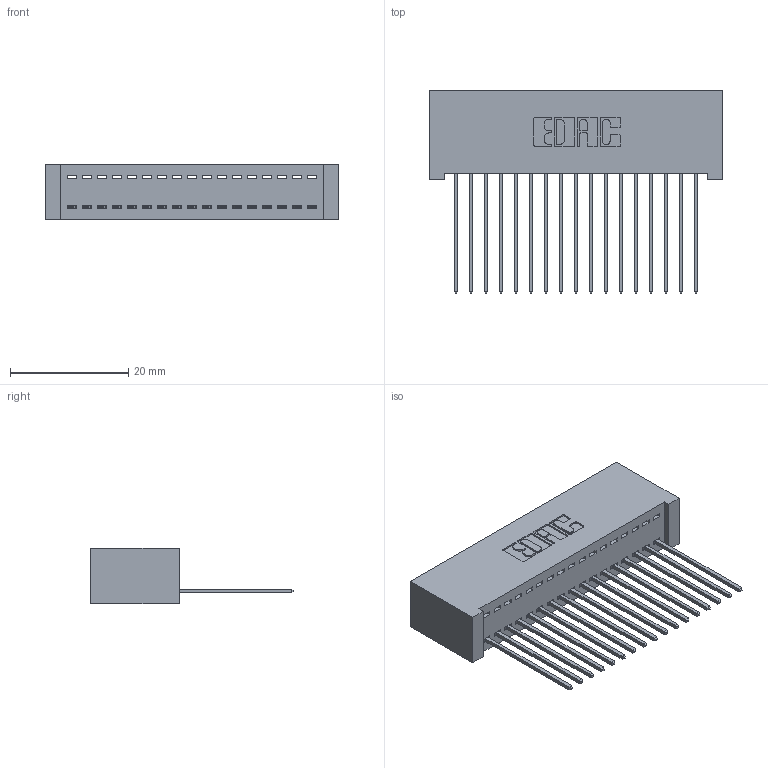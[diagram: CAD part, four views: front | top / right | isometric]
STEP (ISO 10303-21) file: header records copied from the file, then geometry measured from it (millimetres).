
FILE_DESCRIPTION (( 'STEP AP203' ), '1' );
FILE_NAME ('392-017-541-101.STEP', '2019-10-07T03:41:49', ( '' ), ( '' ), 'SwSTEP 2.0', 'SolidWorks 2016', '' );
FILE_SCHEMA (( 'CONFIG_CONTROL_DESIGN' ));
Length unit declared in the file: inch
Products named in the file (3): 342 Part_Lugless; 345-292-001_345-293-141; 392-017-541-101
Assembly tree (18 placements, depth 2):
  392-017-541-101
    342 Part_Lugless
    345-292-001_345-293-141  x17
Bounding box: 49.43 x 34.3 x 9.4 mm (x, y, z)
Volume: 4706.9 mm3; surface area: 7087.3 mm2
Topology: 18 solids, 18 shells, 1088 faces, 3267 edges, 2154 vertices
Faces by surface type: plane 776, cylinder 312
Entity records: 13235 total; most frequent: CARTESIAN_POINT 2293, ORIENTED_EDGE 2246, DIRECTION 1977, EDGE_CURVE 1123, VECTOR 1003, LINE 1003, VERTEX_POINT 746, AXIS2_PLACEMENT_3D 487
